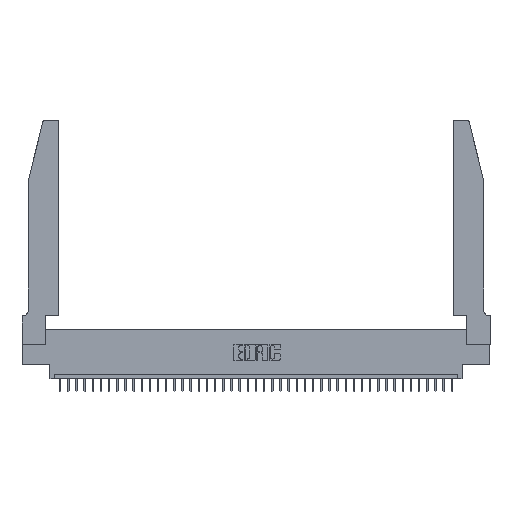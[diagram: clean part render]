
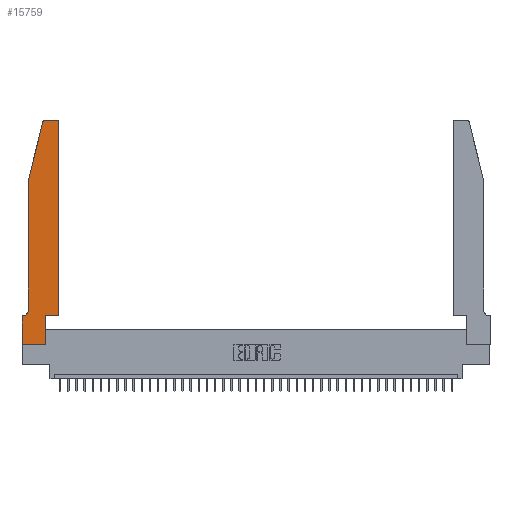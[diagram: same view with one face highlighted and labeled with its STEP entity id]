
A CAD part, top view. The second image highlights one B-rep face of the part: STEP entity #15759.
In plain terms, the highlighted planar face has unit normal (0, 0, 1).
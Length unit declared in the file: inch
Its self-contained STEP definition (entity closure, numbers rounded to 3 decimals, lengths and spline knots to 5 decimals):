
#1026 = LINE ( 'NONE', #2265, #27235 ) ;
#1446 = LINE ( 'NONE', #33147, #16675 ) ;
#2029 = EDGE_CURVE ( 'NONE', #28762, #25634, #7343, .T. ) ;
#2192 = CARTESIAN_POINT ( 'NONE',  ( 0.284, 2.75, 0.37 ) ) ;
#2265 = CARTESIAN_POINT ( 'NONE',  ( 0.0755, 2., 0.37 ) ) ;
#3020 = PLANE ( 'NONE',  #39086 ) ;
#3201 = DIRECTION ( 'NONE',  ( -1., 0., 0. ) ) ;
#3254 = CARTESIAN_POINT ( 'NONE',  ( 0.25487, 2.72718, 0.37 ) ) ;
#3387 = DIRECTION ( 'NONE',  ( 1., 0., 0. ) ) ;
#3569 = CARTESIAN_POINT ( 'NONE',  ( 0., 0.35, 0.37 ) ) ;
#3659 = VECTOR ( 'NONE', #38800, 39.37008 ) ;
#4205 = ORIENTED_EDGE ( 'NONE', *, *, #21367, .T. ) ;
#4437 = VERTEX_POINT ( 'NONE', #26714 ) ;
#4568 = CIRCLE ( 'NONE', #32198, 0.03 ) ;
#5054 = VERTEX_POINT ( 'NONE', #18072 ) ;
#5807 = ORIENTED_EDGE ( 'NONE', *, *, #23881, .T. ) ;
#6033 = DIRECTION ( 'NONE',  ( 1., 0., 0. ) ) ;
#6575 = VERTEX_POINT ( 'NONE', #3254 ) ;
#6627 = LINE ( 'NONE', #30949, #32886 ) ;
#6831 = CARTESIAN_POINT ( 'NONE',  ( 0.2865, 0.35, 0.37 ) ) ;
#7057 = ORIENTED_EDGE ( 'NONE', *, *, #18108, .T. ) ;
#7074 = CARTESIAN_POINT ( 'NONE',  ( 0.4505, 0.35, 0.37 ) ) ;
#7082 = VERTEX_POINT ( 'NONE', #35184 ) ;
#7343 = LINE ( 'NONE', #22497, #31635 ) ;
#8062 = CARTESIAN_POINT ( 'NONE',  ( 0., 0., 0.37 ) ) ;
#9332 = CARTESIAN_POINT ( 'NONE',  ( 0.4205, 2.72, 0.37 ) ) ;
#11025 = EDGE_LOOP ( 'NONE', ( #34778, #26064, #37057, #33009, #7057, #19753, #5807, #40856, #4205, #15346, #32762, #12345 ) ) ;
#11454 = DIRECTION ( 'NONE',  ( 0., 0., -1. ) ) ;
#12039 = LINE ( 'NONE', #8062, #23886 ) ;
#12300 = CARTESIAN_POINT ( 'NONE',  ( 0.2865, 0., 0.37 ) ) ;
#12345 = ORIENTED_EDGE ( 'NONE', *, *, #34928, .T. ) ;
#13387 = DIRECTION ( 'NONE',  ( 1., 0., 0. ) ) ;
#13412 = DIRECTION ( 'NONE',  ( 0., 1., 0. ) ) ;
#13829 = VERTEX_POINT ( 'NONE', #16592 ) ;
#14280 = DIRECTION ( 'NONE',  ( 1., 0., 0. ) ) ;
#14594 = EDGE_CURVE ( 'NONE', #32593, #6575, #4568, .T. ) ;
#15346 = ORIENTED_EDGE ( 'NONE', *, *, #36896, .T. ) ;
#15759 = ADVANCED_FACE ( 'NONE', ( #24313 ), #3020, .T. ) ;
#15783 = DIRECTION ( 'NONE',  ( 0., 0., 1. ) ) ;
#16592 = CARTESIAN_POINT ( 'NONE',  ( 0.0755, 0.42, 0.37 ) ) ;
#16675 = VECTOR ( 'NONE', #36455, 39.37008 ) ;
#16804 = CARTESIAN_POINT ( 'NONE',  ( 0.0755, 2., 0.37 ) ) ;
#18072 = CARTESIAN_POINT ( 'NONE',  ( 0.0755, 2., 0.37 ) ) ;
#18108 = EDGE_CURVE ( 'NONE', #13829, #20215, #22155, .T. ) ;
#18305 = EDGE_CURVE ( 'NONE', #34817, #4437, #1446, .T. ) ;
#18975 = DIRECTION ( 'NONE',  ( 0., -1., 0. ) ) ;
#19753 = ORIENTED_EDGE ( 'NONE', *, *, #31484, .T. ) ;
#20215 = VERTEX_POINT ( 'NONE', #22741 ) ;
#20221 = EDGE_CURVE ( 'NONE', #6575, #5054, #39268, .T. ) ;
#20981 = DIRECTION ( 'NONE',  ( -1., 0., 0. ) ) ;
#21367 = EDGE_CURVE ( 'NONE', #25634, #7082, #33264, .T. ) ;
#22155 = CIRCLE ( 'NONE', #25361, 0.07 ) ;
#22299 = CARTESIAN_POINT ( 'NONE',  ( 0.4205, 2.75, 0.37 ) ) ;
#22497 = CARTESIAN_POINT ( 'NONE',  ( 0., 0., 0.37 ) ) ;
#22741 = CARTESIAN_POINT ( 'NONE',  ( 0.0055, 0.35, 0.37 ) ) ;
#22747 = VECTOR ( 'NONE', #13387, 39.37008 ) ;
#23455 = CIRCLE ( 'NONE', #24217, 0.03 ) ;
#23721 = CARTESIAN_POINT ( 'NONE',  ( 0., 0., 0.37 ) ) ;
#23881 = EDGE_CURVE ( 'NONE', #36150, #28762, #12039, .T. ) ;
#23886 = VECTOR ( 'NONE', #27709, 39.37008 ) ;
#24217 = AXIS2_PLACEMENT_3D ( 'NONE', #9332, #31220, #6033 ) ;
#24313 = FACE_OUTER_BOUND ( 'NONE', #11025, .T. ) ;
#25170 = EDGE_CURVE ( 'NONE', #30544, #32593, #26231, .T. ) ;
#25178 = CARTESIAN_POINT ( 'NONE',  ( 0., 0.35, 0.37 ) ) ;
#25361 = AXIS2_PLACEMENT_3D ( 'NONE', #33465, #11454, #20981 ) ;
#25634 = VERTEX_POINT ( 'NONE', #12300 ) ;
#26064 = ORIENTED_EDGE ( 'NONE', *, *, #14594, .T. ) ;
#26145 = CARTESIAN_POINT ( 'NONE',  ( 0.2605, 2.75, 0.37 ) ) ;
#26231 = LINE ( 'NONE', #26145, #31743 ) ;
#26714 = CARTESIAN_POINT ( 'NONE',  ( 0.4505, 2.72, 0.37 ) ) ;
#27235 = VECTOR ( 'NONE', #18975, 39.37008 ) ;
#27709 = DIRECTION ( 'NONE',  ( 0., -1., 0. ) ) ;
#27743 = CARTESIAN_POINT ( 'NONE',  ( 0.4505, 0.35, 0.37 ) ) ;
#28762 = VERTEX_POINT ( 'NONE', #23721 ) ;
#30544 = VERTEX_POINT ( 'NONE', #22299 ) ;
#30949 = CARTESIAN_POINT ( 'NONE',  ( 0.0755, 0.35, 0.37 ) ) ;
#31078 = DIRECTION ( 'NONE',  ( -1., 0., 0. ) ) ;
#31220 = DIRECTION ( 'NONE',  ( 0., 0., 1. ) ) ;
#31484 = EDGE_CURVE ( 'NONE', #20215, #36150, #6627, .T. ) ;
#31635 = VECTOR ( 'NONE', #3387, 39.37008 ) ;
#31743 = VECTOR ( 'NONE', #3201, 39.37008 ) ;
#31746 = DIRECTION ( 'NONE',  ( 1., 0., 0. ) ) ;
#32198 = AXIS2_PLACEMENT_3D ( 'NONE', #36111, #33234, #14280 ) ;
#32242 = VECTOR ( 'NONE', #13412, 39.37008 ) ;
#32593 = VERTEX_POINT ( 'NONE', #2192 ) ;
#32762 = ORIENTED_EDGE ( 'NONE', *, *, #18305, .T. ) ;
#32886 = VECTOR ( 'NONE', #31078, 39.37008 ) ;
#33009 = ORIENTED_EDGE ( 'NONE', *, *, #37923, .T. ) ;
#33147 = CARTESIAN_POINT ( 'NONE',  ( 0.4505, 0.35, 0.37 ) ) ;
#33222 = LINE ( 'NONE', #7074, #22747 ) ;
#33234 = DIRECTION ( 'NONE',  ( 0., 0., 1. ) ) ;
#33264 = LINE ( 'NONE', #6831, #32242 ) ;
#33465 = CARTESIAN_POINT ( 'NONE',  ( 0.0055, 0.42, 0.37 ) ) ;
#34778 = ORIENTED_EDGE ( 'NONE', *, *, #25170, .T. ) ;
#34817 = VERTEX_POINT ( 'NONE', #27743 ) ;
#34928 = EDGE_CURVE ( 'NONE', #4437, #30544, #23455, .T. ) ;
#35184 = CARTESIAN_POINT ( 'NONE',  ( 0.2865, 0.35, 0.37 ) ) ;
#36111 = CARTESIAN_POINT ( 'NONE',  ( 0.284, 2.72, 0.37 ) ) ;
#36150 = VERTEX_POINT ( 'NONE', #3569 ) ;
#36455 = DIRECTION ( 'NONE',  ( 0., 1., 0. ) ) ;
#36896 = EDGE_CURVE ( 'NONE', #7082, #34817, #33222, .T. ) ;
#37057 = ORIENTED_EDGE ( 'NONE', *, *, #20221, .T. ) ;
#37923 = EDGE_CURVE ( 'NONE', #5054, #13829, #1026, .T. ) ;
#38800 = DIRECTION ( 'NONE',  ( -0.239, -0.971, 0. ) ) ;
#39086 = AXIS2_PLACEMENT_3D ( 'NONE', #25178, #15783, #31746 ) ;
#39268 = LINE ( 'NONE', #16804, #3659 ) ;
#40856 = ORIENTED_EDGE ( 'NONE', *, *, #2029, .T. ) ;
